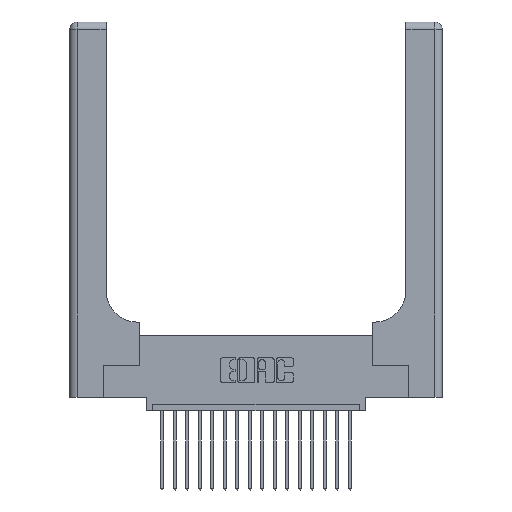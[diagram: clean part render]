
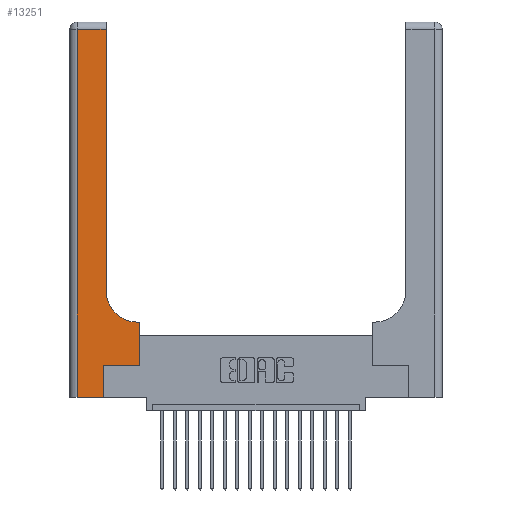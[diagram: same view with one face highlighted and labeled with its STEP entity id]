
A CAD part, top view. The second image highlights one B-rep face of the part: STEP entity #13251.
In plain terms, the highlighted planar face has unit normal (0, 0, 1).
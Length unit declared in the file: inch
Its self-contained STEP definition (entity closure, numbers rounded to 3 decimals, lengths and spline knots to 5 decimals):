
#106 = EDGE_CURVE ( 'NONE', #19854, #3637, #20119, .T. ) ;
#196 = CARTESIAN_POINT ( 'NONE',  ( 0.06, 2.94, 0.37 ) ) ;
#403 = VERTEX_POINT ( 'NONE', #196 ) ;
#760 = CARTESIAN_POINT ( 'NONE',  ( 0., 2.94, 0.37 ) ) ;
#797 = LINE ( 'NONE', #760, #8604 ) ;
#1217 = VERTEX_POINT ( 'NONE', #12777 ) ;
#1518 = LINE ( 'NONE', #5072, #18924 ) ;
#1524 = DIRECTION ( 'NONE',  ( 1., 0., 0. ) ) ;
#1650 = ORIENTED_EDGE ( 'NONE', *, *, #14661, .T. ) ;
#2729 = CARTESIAN_POINT ( 'NONE',  ( 0.269, 0.25, 0.37 ) ) ;
#3415 = EDGE_CURVE ( 'NONE', #1217, #19854, #20388, .T. ) ;
#3543 = DIRECTION ( 'NONE',  ( 0., 0., -1. ) ) ;
#3637 = VERTEX_POINT ( 'NONE', #13601 ) ;
#3939 = CARTESIAN_POINT ( 'NONE',  ( 0.5415, 0.85, 0.37 ) ) ;
#4298 = VERTEX_POINT ( 'NONE', #10774 ) ;
#4646 = VECTOR ( 'NONE', #16958, 39.37008 ) ;
#4794 = ORIENTED_EDGE ( 'NONE', *, *, #12101, .T. ) ;
#5067 = EDGE_CURVE ( 'NONE', #9920, #4298, #20804, .T. ) ;
#5072 = CARTESIAN_POINT ( 'NONE',  ( 0.2915, 0.6, 0.37 ) ) ;
#5341 = DIRECTION ( 'NONE',  ( 1., 0., 0. ) ) ;
#5640 = CARTESIAN_POINT ( 'NONE',  ( 0.06, 3., 0.37 ) ) ;
#5834 = AXIS2_PLACEMENT_3D ( 'NONE', #3939, #19941, #5341 ) ;
#5994 = CARTESIAN_POINT ( 'NONE',  ( 0.5415, 0.6, 0.37 ) ) ;
#6092 = ORIENTED_EDGE ( 'NONE', *, *, #3415, .T. ) ;
#6580 = DIRECTION ( 'NONE',  ( 0., 1., 0. ) ) ;
#8105 = DIRECTION ( 'NONE',  ( -1., 0., 0. ) ) ;
#8131 = EDGE_CURVE ( 'NONE', #14349, #403, #797, .T. ) ;
#8604 = VECTOR ( 'NONE', #15413, 39.37008 ) ;
#8632 = VERTEX_POINT ( 'NONE', #9509 ) ;
#8714 = VECTOR ( 'NONE', #14721, 39.37008 ) ;
#8727 = DIRECTION ( 'NONE',  ( -1., 0., 0. ) ) ;
#9509 = CARTESIAN_POINT ( 'NONE',  ( 0.2915, 0.85, 0.37 ) ) ;
#9770 = CARTESIAN_POINT ( 'NONE',  ( 0.269, 0., 0.37 ) ) ;
#9920 = VERTEX_POINT ( 'NONE', #14245 ) ;
#10630 = DIRECTION ( 'NONE',  ( 1., 0., 0. ) ) ;
#10712 = VECTOR ( 'NONE', #1524, 39.37008 ) ;
#10774 = CARTESIAN_POINT ( 'NONE',  ( 0.269, 0., 0.37 ) ) ;
#11723 = VERTEX_POINT ( 'NONE', #5994 ) ;
#11753 = ORIENTED_EDGE ( 'NONE', *, *, #14226, .T. ) ;
#12038 = VECTOR ( 'NONE', #10630, 39.37008 ) ;
#12101 = EDGE_CURVE ( 'NONE', #3637, #11723, #1518, .T. ) ;
#12110 = ORIENTED_EDGE ( 'NONE', *, *, #19995, .T. ) ;
#12655 = CARTESIAN_POINT ( 'NONE',  ( 0., 0., 0.37 ) ) ;
#12777 = CARTESIAN_POINT ( 'NONE',  ( 0.269, 0.25, 0.37 ) ) ;
#12971 = DIRECTION ( 'NONE',  ( 0., 1., 0. ) ) ;
#13181 = CARTESIAN_POINT ( 'NONE',  ( 0.5585, 0.25, 0.37 ) ) ;
#13251 = ADVANCED_FACE ( 'NONE', ( #17374 ), #18000, .F. ) ;
#13601 = CARTESIAN_POINT ( 'NONE',  ( 0.5585, 0.6, 0.37 ) ) ;
#14226 = EDGE_CURVE ( 'NONE', #11723, #8632, #15298, .T. ) ;
#14245 = CARTESIAN_POINT ( 'NONE',  ( 0.06, 0., 0.37 ) ) ;
#14349 = VERTEX_POINT ( 'NONE', #15516 ) ;
#14571 = ORIENTED_EDGE ( 'NONE', *, *, #8131, .T. ) ;
#14649 = CARTESIAN_POINT ( 'NONE',  ( 0.2915, 3., 0.37 ) ) ;
#14658 = ORIENTED_EDGE ( 'NONE', *, *, #15385, .T. ) ;
#14661 = EDGE_CURVE ( 'NONE', #8632, #14349, #17047, .T. ) ;
#14721 = DIRECTION ( 'NONE',  ( 0., 1., 0. ) ) ;
#15298 = CIRCLE ( 'NONE', #5834, 0.25 ) ;
#15385 = EDGE_CURVE ( 'NONE', #403, #9920, #17019, .T. ) ;
#15413 = DIRECTION ( 'NONE',  ( -1., 0., 0. ) ) ;
#15516 = CARTESIAN_POINT ( 'NONE',  ( 0.2915, 2.94, 0.37 ) ) ;
#15940 = ORIENTED_EDGE ( 'NONE', *, *, #5067, .T. ) ;
#16382 = CARTESIAN_POINT ( 'NONE',  ( 0., 3., 0.37 ) ) ;
#16392 = AXIS2_PLACEMENT_3D ( 'NONE', #16382, #3543, #8105 ) ;
#16958 = DIRECTION ( 'NONE',  ( 0., -1., 0. ) ) ;
#17019 = LINE ( 'NONE', #5640, #4646 ) ;
#17047 = LINE ( 'NONE', #14649, #8714 ) ;
#17346 = EDGE_LOOP ( 'NONE', ( #1650, #14571, #14658, #15940, #12110, #6092, #18128, #4794, #11753 ) ) ;
#17374 = FACE_OUTER_BOUND ( 'NONE', #17346, .T. ) ;
#18000 = PLANE ( 'NONE',  #16392 ) ;
#18128 = ORIENTED_EDGE ( 'NONE', *, *, #106, .T. ) ;
#18651 = VECTOR ( 'NONE', #6580, 39.37008 ) ;
#18924 = VECTOR ( 'NONE', #8727, 39.37008 ) ;
#19612 = VECTOR ( 'NONE', #12971, 39.37008 ) ;
#19854 = VERTEX_POINT ( 'NONE', #20419 ) ;
#19941 = DIRECTION ( 'NONE',  ( 0., 0., -1. ) ) ;
#19995 = EDGE_CURVE ( 'NONE', #4298, #1217, #20412, .T. ) ;
#20119 = LINE ( 'NONE', #13181, #19612 ) ;
#20388 = LINE ( 'NONE', #2729, #12038 ) ;
#20412 = LINE ( 'NONE', #9770, #18651 ) ;
#20419 = CARTESIAN_POINT ( 'NONE',  ( 0.5585, 0.25, 0.37 ) ) ;
#20804 = LINE ( 'NONE', #12655, #10712 ) ;
